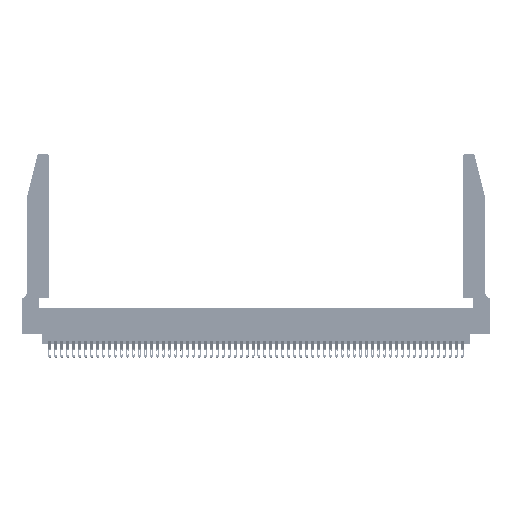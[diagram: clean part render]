
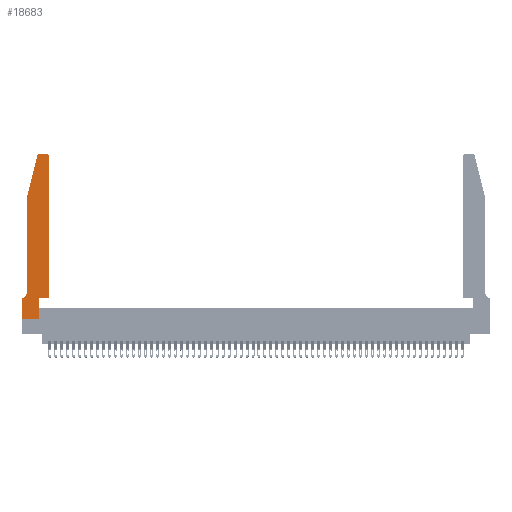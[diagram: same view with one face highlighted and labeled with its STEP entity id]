
A CAD part, top view. The second image highlights one B-rep face of the part: STEP entity #18683.
In plain terms, the highlighted planar face has unit normal (0, 0, 1).
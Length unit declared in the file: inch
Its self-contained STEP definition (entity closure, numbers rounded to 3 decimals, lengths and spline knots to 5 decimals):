
#295 = VECTOR ( 'NONE', #11591, 39.37008 ) ;
#1968 = DIRECTION ( 'NONE',  ( 0., 1., 0. ) ) ;
#2065 = EDGE_CURVE ( 'NONE', #30886, #8452, #16283, .T. ) ;
#2103 = DIRECTION ( 'NONE',  ( 0., 0., 1. ) ) ;
#2142 = DIRECTION ( 'NONE',  ( 1., 0., 0. ) ) ;
#2196 = AXIS2_PLACEMENT_3D ( 'NONE', #15832, #46275, #20232 ) ;
#3995 = EDGE_CURVE ( 'NONE', #11843, #30886, #36644, .T. ) ;
#4536 = CARTESIAN_POINT ( 'NONE',  ( 0.0755, 2., 0.37 ) ) ;
#5033 = FACE_OUTER_BOUND ( 'NONE', #15111, .T. ) ;
#5761 = ORIENTED_EDGE ( 'NONE', *, *, #22259, .T. ) ;
#6385 = ORIENTED_EDGE ( 'NONE', *, *, #23815, .T. ) ;
#8452 = VERTEX_POINT ( 'NONE', #23319 ) ;
#8581 = CARTESIAN_POINT ( 'NONE',  ( 0.2865, 0.35, 0.37 ) ) ;
#8905 = ORIENTED_EDGE ( 'NONE', *, *, #30054, .T. ) ;
#9141 = LINE ( 'NONE', #49828, #42660 ) ;
#10304 = CARTESIAN_POINT ( 'NONE',  ( 0., 0., 0.37 ) ) ;
#11143 = ORIENTED_EDGE ( 'NONE', *, *, #39983, .T. ) ;
#11591 = DIRECTION ( 'NONE',  ( 1., 0., 0. ) ) ;
#11843 = VERTEX_POINT ( 'NONE', #32839 ) ;
#12448 = VERTEX_POINT ( 'NONE', #13406 ) ;
#12567 = LINE ( 'NONE', #50529, #34440 ) ;
#12686 = CIRCLE ( 'NONE', #24264, 0.03 ) ;
#13406 = CARTESIAN_POINT ( 'NONE',  ( 0.284, 2.75, 0.37 ) ) ;
#14003 = CARTESIAN_POINT ( 'NONE',  ( 0., 0.35, 0.37 ) ) ;
#14759 = VERTEX_POINT ( 'NONE', #42348 ) ;
#15006 = VERTEX_POINT ( 'NONE', #30781 ) ;
#15065 = ORIENTED_EDGE ( 'NONE', *, *, #2065, .T. ) ;
#15111 = EDGE_LOOP ( 'NONE', ( #21998, #48915, #8905, #6385, #46087, #24001, #5761, #31708, #15065, #44023, #31895, #11143 ) ) ;
#15723 = CARTESIAN_POINT ( 'NONE',  ( 0.0755, 0.35, 0.37 ) ) ;
#15832 = CARTESIAN_POINT ( 'NONE',  ( 0.0055, 0.42, 0.37 ) ) ;
#16283 = LINE ( 'NONE', #8581, #23822 ) ;
#16638 = VERTEX_POINT ( 'NONE', #41828 ) ;
#17795 = LINE ( 'NONE', #15723, #39614 ) ;
#18218 = LINE ( 'NONE', #10304, #28514 ) ;
#18435 = DIRECTION ( 'NONE',  ( 1., 0., 0. ) ) ;
#18683 = ADVANCED_FACE ( 'NONE', ( #5033 ), #40144, .T. ) ;
#19194 = CIRCLE ( 'NONE', #2196, 0.07 ) ;
#19851 = CARTESIAN_POINT ( 'NONE',  ( 0., 0.35, 0.37 ) ) ;
#20232 = DIRECTION ( 'NONE',  ( -1., 0., 0. ) ) ;
#21129 = LINE ( 'NONE', #4536, #32787 ) ;
#21852 = DIRECTION ( 'NONE',  ( -1., 0., 0. ) ) ;
#21998 = ORIENTED_EDGE ( 'NONE', *, *, #48346, .T. ) ;
#22259 = EDGE_CURVE ( 'NONE', #46264, #11843, #18218, .T. ) ;
#22677 = LINE ( 'NONE', #51841, #32952 ) ;
#23319 = CARTESIAN_POINT ( 'NONE',  ( 0.2865, 0.35, 0.37 ) ) ;
#23652 = AXIS2_PLACEMENT_3D ( 'NONE', #14003, #44460, #18435 ) ;
#23815 = EDGE_CURVE ( 'NONE', #14759, #15006, #12567, .T. ) ;
#23822 = VECTOR ( 'NONE', #34647, 39.37008 ) ;
#24001 = ORIENTED_EDGE ( 'NONE', *, *, #56032, .T. ) ;
#24264 = AXIS2_PLACEMENT_3D ( 'NONE', #28401, #2103, #32793 ) ;
#25478 = VERTEX_POINT ( 'NONE', #44707 ) ;
#25804 = CIRCLE ( 'NONE', #50873, 0.03 ) ;
#25881 = EDGE_CURVE ( 'NONE', #8452, #48359, #22677, .T. ) ;
#28401 = CARTESIAN_POINT ( 'NONE',  ( 0.4205, 2.72, 0.37 ) ) ;
#28444 = DIRECTION ( 'NONE',  ( 0., 0., 1. ) ) ;
#28514 = VECTOR ( 'NONE', #40861, 39.37008 ) ;
#30054 = EDGE_CURVE ( 'NONE', #39773, #14759, #21129, .T. ) ;
#30310 = DIRECTION ( 'NONE',  ( 1., 0., 0. ) ) ;
#30781 = CARTESIAN_POINT ( 'NONE',  ( 0.0755, 0.42, 0.37 ) ) ;
#30886 = VERTEX_POINT ( 'NONE', #40197 ) ;
#31054 = EDGE_CURVE ( 'NONE', #12448, #39773, #25804, .T. ) ;
#31708 = ORIENTED_EDGE ( 'NONE', *, *, #3995, .T. ) ;
#31895 = ORIENTED_EDGE ( 'NONE', *, *, #33028, .T. ) ;
#32787 = VECTOR ( 'NONE', #35163, 39.37008 ) ;
#32793 = DIRECTION ( 'NONE',  ( 1., 0., 0. ) ) ;
#32839 = CARTESIAN_POINT ( 'NONE',  ( 0., 0., 0.37 ) ) ;
#32952 = VECTOR ( 'NONE', #30310, 39.37008 ) ;
#33028 = EDGE_CURVE ( 'NONE', #48359, #42652, #9141, .T. ) ;
#34440 = VECTOR ( 'NONE', #54839, 39.37008 ) ;
#34647 = DIRECTION ( 'NONE',  ( 0., 1., 0. ) ) ;
#34996 = CARTESIAN_POINT ( 'NONE',  ( 0.4505, 0.35, 0.37 ) ) ;
#35163 = DIRECTION ( 'NONE',  ( -0.239, -0.971, 0. ) ) ;
#35802 = CARTESIAN_POINT ( 'NONE',  ( 0.25487, 2.72718, 0.37 ) ) ;
#36133 = LINE ( 'NONE', #39182, #56339 ) ;
#36644 = LINE ( 'NONE', #37759, #295 ) ;
#37759 = CARTESIAN_POINT ( 'NONE',  ( 0., 0., 0.37 ) ) ;
#39182 = CARTESIAN_POINT ( 'NONE',  ( 0.2605, 2.75, 0.37 ) ) ;
#39614 = VECTOR ( 'NONE', #41638, 39.37008 ) ;
#39773 = VERTEX_POINT ( 'NONE', #35802 ) ;
#39983 = EDGE_CURVE ( 'NONE', #42652, #16638, #12686, .T. ) ;
#40144 = PLANE ( 'NONE',  #23652 ) ;
#40197 = CARTESIAN_POINT ( 'NONE',  ( 0.2865, 0., 0.37 ) ) ;
#40861 = DIRECTION ( 'NONE',  ( 0., -1., 0. ) ) ;
#41327 = EDGE_CURVE ( 'NONE', #15006, #25478, #19194, .T. ) ;
#41638 = DIRECTION ( 'NONE',  ( -1., 0., 0. ) ) ;
#41828 = CARTESIAN_POINT ( 'NONE',  ( 0.4205, 2.75, 0.37 ) ) ;
#42348 = CARTESIAN_POINT ( 'NONE',  ( 0.0755, 2., 0.37 ) ) ;
#42652 = VERTEX_POINT ( 'NONE', #48629 ) ;
#42660 = VECTOR ( 'NONE', #1968, 39.37008 ) ;
#44023 = ORIENTED_EDGE ( 'NONE', *, *, #25881, .T. ) ;
#44460 = DIRECTION ( 'NONE',  ( 0., 0., 1. ) ) ;
#44707 = CARTESIAN_POINT ( 'NONE',  ( 0.0055, 0.35, 0.37 ) ) ;
#46087 = ORIENTED_EDGE ( 'NONE', *, *, #41327, .T. ) ;
#46264 = VERTEX_POINT ( 'NONE', #19851 ) ;
#46275 = DIRECTION ( 'NONE',  ( 0., 0., -1. ) ) ;
#48346 = EDGE_CURVE ( 'NONE', #16638, #12448, #36133, .T. ) ;
#48359 = VERTEX_POINT ( 'NONE', #34996 ) ;
#48629 = CARTESIAN_POINT ( 'NONE',  ( 0.4505, 2.72, 0.37 ) ) ;
#48915 = ORIENTED_EDGE ( 'NONE', *, *, #31054, .T. ) ;
#49828 = CARTESIAN_POINT ( 'NONE',  ( 0.4505, 0.35, 0.37 ) ) ;
#50529 = CARTESIAN_POINT ( 'NONE',  ( 0.0755, 2., 0.37 ) ) ;
#50873 = AXIS2_PLACEMENT_3D ( 'NONE', #54334, #28444, #2142 ) ;
#51841 = CARTESIAN_POINT ( 'NONE',  ( 0.4505, 0.35, 0.37 ) ) ;
#54334 = CARTESIAN_POINT ( 'NONE',  ( 0.284, 2.72, 0.37 ) ) ;
#54839 = DIRECTION ( 'NONE',  ( 0., -1., 0. ) ) ;
#56032 = EDGE_CURVE ( 'NONE', #25478, #46264, #17795, .T. ) ;
#56339 = VECTOR ( 'NONE', #21852, 39.37008 ) ;
